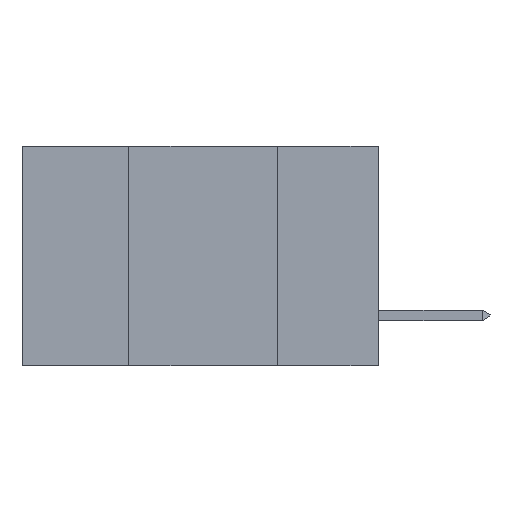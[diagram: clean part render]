
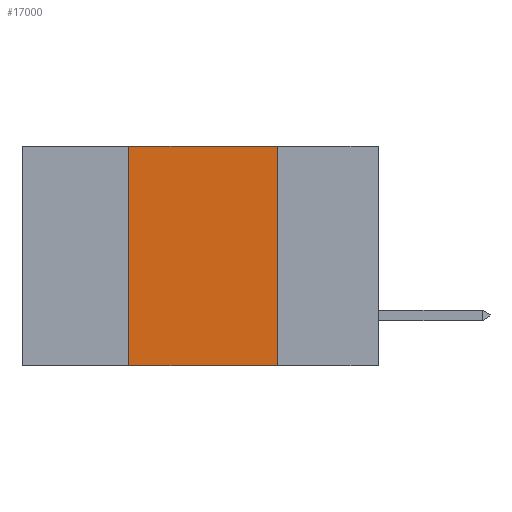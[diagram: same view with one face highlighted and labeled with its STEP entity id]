
A CAD part, left-side view. The second image highlights one B-rep face of the part: STEP entity #17000.
In plain terms, the highlighted planar face has unit normal (-1, 0, 0).
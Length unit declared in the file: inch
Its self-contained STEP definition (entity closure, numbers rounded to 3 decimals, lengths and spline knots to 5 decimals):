
#343 = FACE_OUTER_BOUND ( 'NONE', #13844, .T. ) ;
#1490 = CARTESIAN_POINT ( 'NONE',  ( 0., 0.42, -0.37 ) ) ;
#1606 = DIRECTION ( 'NONE',  ( 0., -1., 0. ) ) ;
#1999 = ORIENTED_EDGE ( 'NONE', *, *, #2475, .F. ) ;
#2475 = EDGE_CURVE ( 'NONE', #12201, #4274, #7317, .T. ) ;
#2764 = CARTESIAN_POINT ( 'NONE',  ( 0., 0.6, -0.37 ) ) ;
#2855 = VECTOR ( 'NONE', #8313, 39.37008 ) ;
#3370 = EDGE_CURVE ( 'NONE', #15437, #14715, #12617, .T. ) ;
#4274 = VERTEX_POINT ( 'NONE', #6330 ) ;
#4642 = ORIENTED_EDGE ( 'NONE', *, *, #8777, .F. ) ;
#5760 = CARTESIAN_POINT ( 'NONE',  ( 0., 0.6, 0. ) ) ;
#5832 = DIRECTION ( 'NONE',  ( 1., 0., 0. ) ) ;
#6109 = CARTESIAN_POINT ( 'NONE',  ( 0., 0.17, 0. ) ) ;
#6330 = CARTESIAN_POINT ( 'NONE',  ( 0., 0.42, 0. ) ) ;
#7292 = CARTESIAN_POINT ( 'NONE',  ( 0., 0.17, -0.37 ) ) ;
#7317 = LINE ( 'NONE', #13544, #2855 ) ;
#7416 = CARTESIAN_POINT ( 'NONE',  ( 0., 0.17, 0. ) ) ;
#8313 = DIRECTION ( 'NONE',  ( 0., 0., 1. ) ) ;
#8584 = ORIENTED_EDGE ( 'NONE', *, *, #3370, .F. ) ;
#8777 = EDGE_CURVE ( 'NONE', #4274, #15437, #11765, .T. ) ;
#10072 = EDGE_CURVE ( 'NONE', #12201, #14715, #16882, .T. ) ;
#10773 = ORIENTED_EDGE ( 'NONE', *, *, #10072, .T. ) ;
#11267 = VECTOR ( 'NONE', #16228, 39.37008 ) ;
#11360 = PLANE ( 'NONE',  #12459 ) ;
#11670 = DIRECTION ( 'NONE',  ( 0., -1., 0. ) ) ;
#11765 = LINE ( 'NONE', #5760, #14891 ) ;
#12201 = VERTEX_POINT ( 'NONE', #1490 ) ;
#12459 = AXIS2_PLACEMENT_3D ( 'NONE', #12803, #5832, #14243 ) ;
#12617 = LINE ( 'NONE', #6109, #11267 ) ;
#12803 = CARTESIAN_POINT ( 'NONE',  ( 0., 0.6, 0. ) ) ;
#13544 = CARTESIAN_POINT ( 'NONE',  ( 0., 0.42, 0. ) ) ;
#13844 = EDGE_LOOP ( 'NONE', ( #8584, #4642, #1999, #10773 ) ) ;
#14243 = DIRECTION ( 'NONE',  ( 0., 0., -1. ) ) ;
#14616 = VECTOR ( 'NONE', #11670, 39.37008 ) ;
#14715 = VERTEX_POINT ( 'NONE', #7292 ) ;
#14891 = VECTOR ( 'NONE', #1606, 39.37008 ) ;
#15437 = VERTEX_POINT ( 'NONE', #7416 ) ;
#16228 = DIRECTION ( 'NONE',  ( 0., 0., -1. ) ) ;
#16882 = LINE ( 'NONE', #2764, #14616 ) ;
#17000 = ADVANCED_FACE ( 'NONE', ( #343 ), #11360, .F. ) ;
